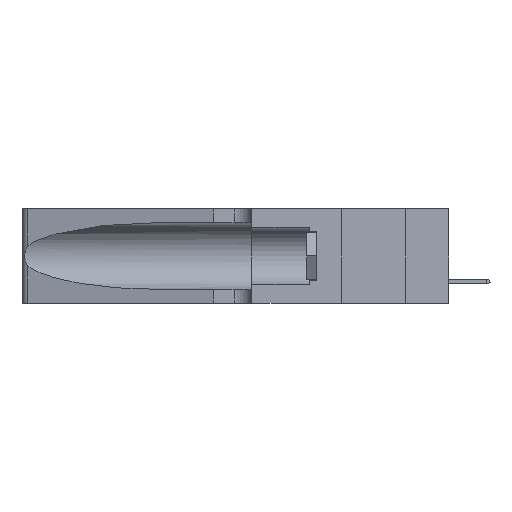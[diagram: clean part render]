
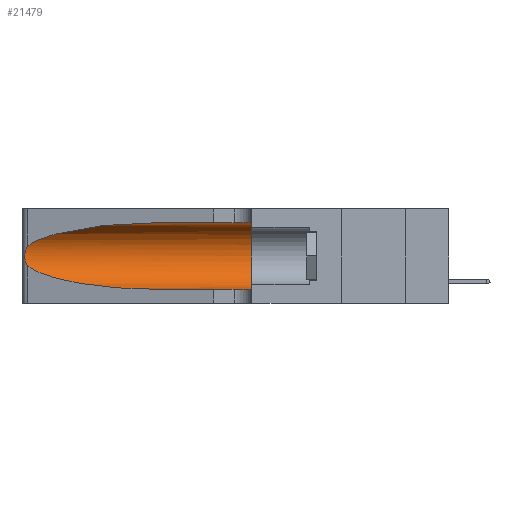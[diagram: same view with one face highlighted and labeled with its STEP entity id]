
A CAD part, left-side view. The second image highlights one B-rep face of the part: STEP entity #21479.
In plain terms, the highlighted cylindrical face has radius 3.308 mm (diameter 6.617 mm), a partial arc.
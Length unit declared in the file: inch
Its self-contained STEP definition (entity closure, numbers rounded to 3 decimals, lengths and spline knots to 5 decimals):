
#1189 = LINE ( 'NONE', #21071, #31524 ) ;
#2052 = ORIENTED_EDGE ( 'NONE', *, *, #45725, .F. ) ;
#3546 = CARTESIAN_POINT ( 'NONE',  ( 0.1305, 0.72297, 0.05475 ) ) ;
#3838 = CARTESIAN_POINT ( 'NONE',  ( 0.25787, 1.23484, 0.2124 ) ) ;
#4058 = VERTEX_POINT ( 'NONE', #10930 ) ;
#4336 = CARTESIAN_POINT ( 'NONE',  ( 0.26017, 1.23833, 0.17102 ) ) ;
#5464 = DIRECTION ( 'NONE',  ( 0., -1., 0. ) ) ;
#6374 = CARTESIAN_POINT ( 'NONE',  ( 0.25856, 1.23593, 0.16098 ) ) ;
#6444 = CARTESIAN_POINT ( 'NONE',  ( 0.25555, 1.22994, 0.2215 ) ) ;
#7551 = EDGE_CURVE ( 'NONE', #46661, #47365, #40794, .T. ) ;
#7700 = CARTESIAN_POINT ( 'NONE',  ( 0.26018, 1.23835, 0.19895 ) ) ;
#8068 = CARTESIAN_POINT ( 'NONE',  ( 0.25789, 1.23486, 0.15765 ) ) ;
#8267 = LINE ( 'NONE', #45854, #49590 ) ;
#8910 = VERTEX_POINT ( 'NONE', #11271 ) ;
#9233 = DIRECTION ( 'NONE',  ( 0., -1., 0. ) ) ;
#10930 = CARTESIAN_POINT ( 'NONE',  ( 0.1305, 0.35, 0.31525 ) ) ;
#11271 = CARTESIAN_POINT ( 'NONE',  ( 0.1305, 0.72297, 0.31525 ) ) ;
#11384 = CARTESIAN_POINT ( 'NONE',  ( 0.25854, 1.2359, 0.20912 ) ) ;
#11448 = ORIENTED_EDGE ( 'NONE', *, *, #44749, .F. ) ;
#12163 = ORIENTED_EDGE ( 'NONE', *, *, #27757, .T. ) ;
#12971 = CARTESIAN_POINT ( 'NONE',  ( 0.25555, 1.22993, 0.14849 ) ) ;
#13086 = CYLINDRICAL_SURFACE ( 'NONE', #17182, 0.13025 ) ;
#14715 = ORIENTED_EDGE ( 'NONE', *, *, #33302, .T. ) ;
#16564 = CARTESIAN_POINT ( 'NONE',  ( 0.26075, 1.23896, 0.19203 ) ) ;
#17043 = CARTESIAN_POINT ( 'NONE',  ( 0.1305, 0.35, 0.05475 ) ) ;
#17182 = AXIS2_PLACEMENT_3D ( 'NONE', #46232, #42429, #35460 ) ;
#17391 = CARTESIAN_POINT ( 'NONE',  ( 0.1305, 0.72297, 0.31525 ) ) ;
#19009 = CARTESIAN_POINT ( 'NONE',  ( 0.1305, 0.35, 0.185 ) ) ;
#20130 = ORIENTED_EDGE ( 'NONE', *, *, #7551, .T. ) ;
#20697 = FACE_OUTER_BOUND ( 'NONE', #40438, .T. ) ;
#21071 = CARTESIAN_POINT ( 'NONE',  ( 0.1305, 1.61858, 0.31525 ) ) ;
#21479 = ADVANCED_FACE ( 'NONE', ( #20697 ), #13086, .F. ) ;
#22270 = CARTESIAN_POINT ( 'NONE',  ( 0.1305, 0.72297, 0.05475 ) ) ;
#23115 = CARTESIAN_POINT ( 'NONE',  ( 0.25639, 1.23184, 0.21858 ) ) ;
#27097 = CARTESIAN_POINT ( 'NONE',  ( 0.25487, 1.22718, 0.14631 ) ) ;
#27757 = EDGE_CURVE ( 'NONE', #30902, #46661, #41409, .T. ) ;
#29114 = CARTESIAN_POINT ( 'NONE',  ( 0.25487, 1.22718, 0.14631 ) ) ;
#30902 = VERTEX_POINT ( 'NONE', #37031 ) ;
#31524 = VECTOR ( 'NONE', #5464, 39.37008 ) ;
#32243 = CARTESIAN_POINT ( 'NONE',  ( 0.26075, 1.23896, 0.178 ) ) ;
#32294 = CIRCLE ( 'NONE', #45723, 0.13025 ) ;
#33302 = EDGE_CURVE ( 'NONE', #8910, #30902, #46951, .T. ) ;
#35460 = DIRECTION ( 'NONE',  ( 0., 0., -1. ) ) ;
#35802 = CARTESIAN_POINT ( 'NONE',  ( 0.2373, 1.15595, 0.08982 ) ) ;
#37031 = CARTESIAN_POINT ( 'NONE',  ( 0.25487, 1.22718, 0.22369 ) ) ;
#37243 = CARTESIAN_POINT ( 'NONE',  ( 0.25639, 1.23186, 0.15144 ) ) ;
#37501 = CARTESIAN_POINT ( 'NONE',  ( 0.2373, 1.15595, 0.28018 ) ) ;
#38912 = CARTESIAN_POINT ( 'NONE',  ( 0.25487, 1.22718, 0.22369 ) ) ;
#39809 = CARTESIAN_POINT ( 'NONE',  ( 0.18966, 0.96281, 0.05475 ) ) ;
#40438 = EDGE_LOOP ( 'NONE', ( #14715, #12163, #20130, #44741, #11448, #2052 ) ) ;
#40794 =( BOUNDED_CURVE ( )  B_SPLINE_CURVE ( 3, ( #51564, #35802, #39809, #3546 ),
 .UNSPECIFIED., .F., .F. ) 
 B_SPLINE_CURVE_WITH_KNOTS ( ( 4, 4 ),
 ( 3.44316, 4.71239 ),
 .UNSPECIFIED. ) 
 CURVE ( )  GEOMETRIC_REPRESENTATION_ITEM ( )  RATIONAL_B_SPLINE_CURVE ( ( 1., 0.87, 0.87, 1. ) ) 
 REPRESENTATION_ITEM ( '' )  );
#41353 = CARTESIAN_POINT ( 'NONE',  ( 0.25487, 1.22718, 0.22369 ) ) ;
#41409 = B_SPLINE_CURVE_WITH_KNOTS ( 'NONE', 3,
 ( #38912, #6444, #23115, #3838, #11384, #7700, #16564, #32243, #4336, #6374, #8068, #37243, #12971, #29114 ),
 .UNSPECIFIED., .F., .F.,
 ( 4, 2, 2, 2, 2, 2, 4 ),
 ( 0., 0.00027, 0.00053, 0.00107, 0.0016, 0.00187, 0.00214 ),
 .UNSPECIFIED. ) ;
#41709 = EDGE_CURVE ( 'NONE', #47365, #43988, #8267, .T. ) ;
#42429 = DIRECTION ( 'NONE',  ( 0., -1., 0. ) ) ;
#43372 = DIRECTION ( 'NONE',  ( 0., 1., 0. ) ) ;
#43988 = VERTEX_POINT ( 'NONE', #17043 ) ;
#44741 = ORIENTED_EDGE ( 'NONE', *, *, #41709, .T. ) ;
#44749 = EDGE_CURVE ( 'NONE', #4058, #43988, #32294, .T. ) ;
#45417 = CARTESIAN_POINT ( 'NONE',  ( 0.18966, 0.96281, 0.31525 ) ) ;
#45723 = AXIS2_PLACEMENT_3D ( 'NONE', #19009, #43372, #50886 ) ;
#45725 = EDGE_CURVE ( 'NONE', #8910, #4058, #1189, .T. ) ;
#45854 = CARTESIAN_POINT ( 'NONE',  ( 0.1305, 1.61858, 0.05475 ) ) ;
#46232 = CARTESIAN_POINT ( 'NONE',  ( 0.1305, 1.61858, 0.185 ) ) ;
#46661 = VERTEX_POINT ( 'NONE', #27097 ) ;
#46951 =( BOUNDED_CURVE ( )  B_SPLINE_CURVE ( 3, ( #17391, #45417, #37501, #41353 ),
 .UNSPECIFIED., .F., .T. ) 
 B_SPLINE_CURVE_WITH_KNOTS ( ( 4, 4 ),
 ( 1.5708, 2.84003 ),
 .UNSPECIFIED. ) 
 CURVE ( )  GEOMETRIC_REPRESENTATION_ITEM ( )  RATIONAL_B_SPLINE_CURVE ( ( 1., 0.87, 0.87, 1. ) ) 
 REPRESENTATION_ITEM ( '' )  );
#47365 = VERTEX_POINT ( 'NONE', #22270 ) ;
#49590 = VECTOR ( 'NONE', #9233, 39.37008 ) ;
#50886 = DIRECTION ( 'NONE',  ( 0., 0., 1. ) ) ;
#51564 = CARTESIAN_POINT ( 'NONE',  ( 0.25487, 1.22718, 0.14631 ) ) ;
